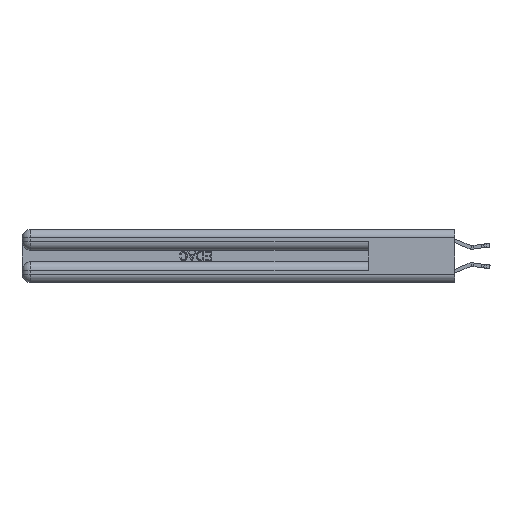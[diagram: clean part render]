
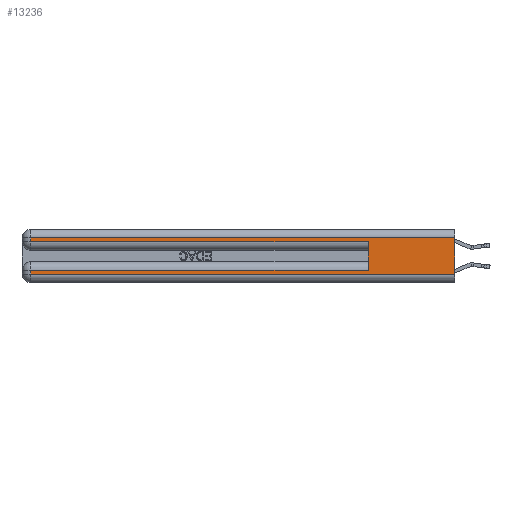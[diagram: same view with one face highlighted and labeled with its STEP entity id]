
A CAD part, left-side view. The second image highlights one B-rep face of the part: STEP entity #13236.
In plain terms, the highlighted planar face has unit normal (-1, 0, 0).
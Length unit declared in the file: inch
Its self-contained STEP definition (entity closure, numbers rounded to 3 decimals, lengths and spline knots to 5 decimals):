
#728 = EDGE_CURVE ( 'NONE', #9642, #34642, #18508, .T. ) ;
#937 = VERTEX_POINT ( 'NONE', #30863 ) ;
#985 = CARTESIAN_POINT ( 'NONE',  ( 0., 0., 0.285 ) ) ;
#1143 = ORIENTED_EDGE ( 'NONE', *, *, #14315, .T. ) ;
#4793 = VECTOR ( 'NONE', #31643, 39.37008 ) ;
#4916 = EDGE_CURVE ( 'NONE', #8068, #11466, #33023, .T. ) ;
#5048 = EDGE_CURVE ( 'NONE', #25130, #11466, #20322, .T. ) ;
#5224 = CARTESIAN_POINT ( 'NONE',  ( 0., 2.94, 0.37 ) ) ;
#5757 = LINE ( 'NONE', #11408, #25612 ) ;
#5942 = CARTESIAN_POINT ( 'NONE',  ( 0., 0.6, 0.145 ) ) ;
#6324 = CARTESIAN_POINT ( 'NONE',  ( 0., 0., 0.06 ) ) ;
#7949 = DIRECTION ( 'NONE',  ( 0., 0., -1. ) ) ;
#8030 = LINE ( 'NONE', #21493, #16461 ) ;
#8068 = VERTEX_POINT ( 'NONE', #33851 ) ;
#9010 = CARTESIAN_POINT ( 'NONE',  ( 0., 0., 0.06 ) ) ;
#9026 = DIRECTION ( 'NONE',  ( 0., 0., 1. ) ) ;
#9238 = FACE_OUTER_BOUND ( 'NONE', #31734, .T. ) ;
#9642 = VERTEX_POINT ( 'NONE', #34690 ) ;
#9909 = CARTESIAN_POINT ( 'NONE',  ( 0., 2.94, 0.285 ) ) ;
#10560 = ORIENTED_EDGE ( 'NONE', *, *, #15303, .T. ) ;
#11408 = CARTESIAN_POINT ( 'NONE',  ( 0., 0., 0.31 ) ) ;
#11466 = VERTEX_POINT ( 'NONE', #21536 ) ;
#11728 = ORIENTED_EDGE ( 'NONE', *, *, #728, .T. ) ;
#12328 = VECTOR ( 'NONE', #20694, 39.37008 ) ;
#12420 = DIRECTION ( 'NONE',  ( 0., -1., 0. ) ) ;
#13236 = ADVANCED_FACE ( 'NONE', ( #9238 ), #26618, .F. ) ;
#13373 = EDGE_CURVE ( 'NONE', #29591, #25130, #33343, .T. ) ;
#14166 = ORIENTED_EDGE ( 'NONE', *, *, #5048, .T. ) ;
#14315 = EDGE_CURVE ( 'NONE', #27602, #29591, #5757, .T. ) ;
#15303 = EDGE_CURVE ( 'NONE', #8068, #937, #30545, .T. ) ;
#15882 = ORIENTED_EDGE ( 'NONE', *, *, #18450, .F. ) ;
#16461 = VECTOR ( 'NONE', #31918, 39.37008 ) ;
#17781 = VECTOR ( 'NONE', #9026, 39.37008 ) ;
#18450 = EDGE_CURVE ( 'NONE', #27602, #34642, #24199, .T. ) ;
#18508 = LINE ( 'NONE', #9010, #29517 ) ;
#19851 = AXIS2_PLACEMENT_3D ( 'NONE', #21043, #29344, #23988 ) ;
#20322 = LINE ( 'NONE', #985, #21606 ) ;
#20382 = DIRECTION ( 'NONE',  ( 0., -1., 0. ) ) ;
#20694 = DIRECTION ( 'NONE',  ( 0., 1., 0. ) ) ;
#21043 = CARTESIAN_POINT ( 'NONE',  ( 0., 0., 0.37 ) ) ;
#21334 = EDGE_CURVE ( 'NONE', #937, #9642, #8030, .T. ) ;
#21493 = CARTESIAN_POINT ( 'NONE',  ( 0., 2.94, 0.37 ) ) ;
#21536 = CARTESIAN_POINT ( 'NONE',  ( 0., 0.6, 0.285 ) ) ;
#21606 = VECTOR ( 'NONE', #20382, 39.37008 ) ;
#23430 = CARTESIAN_POINT ( 'NONE',  ( 0., 0., 0.31 ) ) ;
#23988 = DIRECTION ( 'NONE',  ( 0., 0., -1. ) ) ;
#24199 = LINE ( 'NONE', #28935, #4793 ) ;
#25130 = VERTEX_POINT ( 'NONE', #9909 ) ;
#25612 = VECTOR ( 'NONE', #30681, 39.37008 ) ;
#26374 = CARTESIAN_POINT ( 'NONE',  ( 0., 0., 0.085 ) ) ;
#26618 = PLANE ( 'NONE',  #19851 ) ;
#27602 = VERTEX_POINT ( 'NONE', #23430 ) ;
#28661 = ORIENTED_EDGE ( 'NONE', *, *, #13373, .T. ) ;
#28935 = CARTESIAN_POINT ( 'NONE',  ( 0., 0., 0.37 ) ) ;
#29344 = DIRECTION ( 'NONE',  ( 1., 0., 0. ) ) ;
#29517 = VECTOR ( 'NONE', #12420, 39.37008 ) ;
#29591 = VERTEX_POINT ( 'NONE', #33122 ) ;
#30161 = ORIENTED_EDGE ( 'NONE', *, *, #21334, .T. ) ;
#30545 = LINE ( 'NONE', #26374, #12328 ) ;
#30681 = DIRECTION ( 'NONE',  ( 0., 1., 0. ) ) ;
#30863 = CARTESIAN_POINT ( 'NONE',  ( 0., 2.94, 0.085 ) ) ;
#30998 = ORIENTED_EDGE ( 'NONE', *, *, #4916, .F. ) ;
#31643 = DIRECTION ( 'NONE',  ( 0., 0., -1. ) ) ;
#31734 = EDGE_LOOP ( 'NONE', ( #15882, #1143, #28661, #14166, #30998, #10560, #30161, #11728 ) ) ;
#31918 = DIRECTION ( 'NONE',  ( 0., 0., -1. ) ) ;
#33023 = LINE ( 'NONE', #5942, #17781 ) ;
#33122 = CARTESIAN_POINT ( 'NONE',  ( 0., 2.94, 0.31 ) ) ;
#33343 = LINE ( 'NONE', #5224, #33749 ) ;
#33749 = VECTOR ( 'NONE', #7949, 39.37008 ) ;
#33851 = CARTESIAN_POINT ( 'NONE',  ( 0., 0.6, 0.085 ) ) ;
#34642 = VERTEX_POINT ( 'NONE', #6324 ) ;
#34690 = CARTESIAN_POINT ( 'NONE',  ( 0., 2.94, 0.06 ) ) ;
